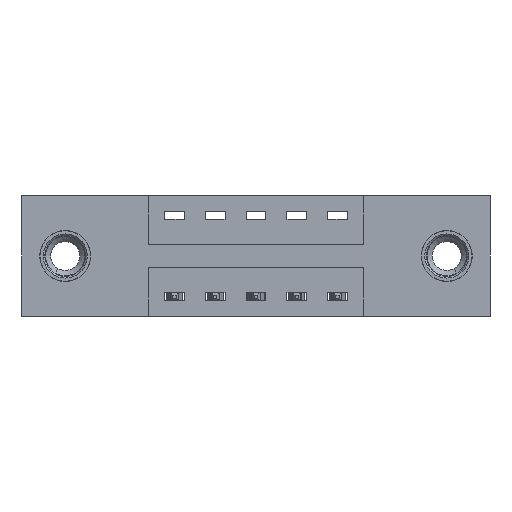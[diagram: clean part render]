
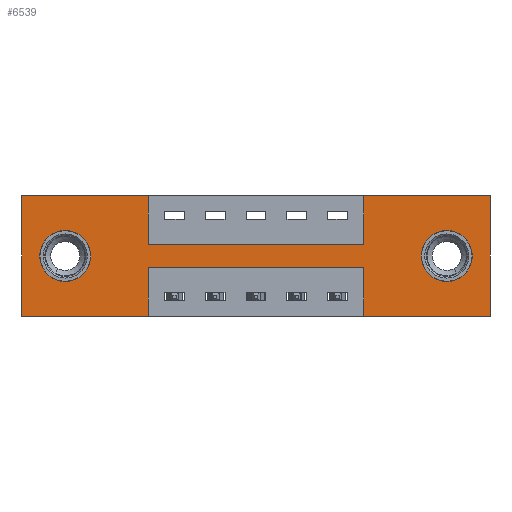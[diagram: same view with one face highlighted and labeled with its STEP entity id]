
A CAD part, front view. The second image highlights one B-rep face of the part: STEP entity #6539.
In plain terms, the highlighted planar face has unit normal (0, -1, 0).
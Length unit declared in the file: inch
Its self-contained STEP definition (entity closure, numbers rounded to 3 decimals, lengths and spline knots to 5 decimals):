
#58 = DIRECTION ( 'NONE',  ( 0., 1., 0. ) ) ;
#68 = LINE ( 'NONE', #8705, #10293 ) ;
#119 = VERTEX_POINT ( 'NONE', #5706 ) ;
#199 = ORIENTED_EDGE ( 'NONE', *, *, #5294, .T. ) ;
#257 = CIRCLE ( 'NONE', #3905, 0.078 ) ;
#302 = LINE ( 'NONE', #12804, #4380 ) ;
#514 = CIRCLE ( 'NONE', #6808, 0.078 ) ;
#545 = CARTESIAN_POINT ( 'NONE',  ( 0.3875, 0., -0.15 ) ) ;
#582 = EDGE_CURVE ( 'NONE', #119, #5072, #11572, .T. ) ;
#781 = VERTEX_POINT ( 'NONE', #3629 ) ;
#917 = CARTESIAN_POINT ( 'NONE',  ( 0.3875, 0., -0.15 ) ) ;
#975 = VECTOR ( 'NONE', #1886, 39.37008 ) ;
#1065 = VECTOR ( 'NONE', #10055, 39.37008 ) ;
#1067 = PLANE ( 'NONE',  #12464 ) ;
#1289 = LINE ( 'NONE', #8876, #2550 ) ;
#1296 = VERTEX_POINT ( 'NONE', #917 ) ;
#1305 = CARTESIAN_POINT ( 'NONE',  ( 0.3875, 0., 0. ) ) ;
#1380 = EDGE_LOOP ( 'NONE', ( #10732, #6123 ) ) ;
#1433 = ORIENTED_EDGE ( 'NONE', *, *, #582, .F. ) ;
#1445 = CARTESIAN_POINT ( 'NONE',  ( 1.3025, 0., -0.107 ) ) ;
#1469 = DIRECTION ( 'NONE',  ( 1., 0., 0. ) ) ;
#1517 = VERTEX_POINT ( 'NONE', #2110 ) ;
#1704 = CARTESIAN_POINT ( 'NONE',  ( 0., 0., 0. ) ) ;
#1751 = VECTOR ( 'NONE', #12090, 39.37008 ) ;
#1886 = DIRECTION ( 'NONE',  ( -1., 0., 0. ) ) ;
#1966 = ORIENTED_EDGE ( 'NONE', *, *, #2971, .F. ) ;
#1979 = CARTESIAN_POINT ( 'NONE',  ( 1.0475, 0., -0.15 ) ) ;
#2042 = VECTOR ( 'NONE', #8438, 39.37008 ) ;
#2110 = CARTESIAN_POINT ( 'NONE',  ( 1.3025, 0., -0.263 ) ) ;
#2323 = LINE ( 'NONE', #7987, #1065 ) ;
#2514 = LINE ( 'NONE', #545, #4100 ) ;
#2535 = VECTOR ( 'NONE', #4720, 39.37008 ) ;
#2550 = VECTOR ( 'NONE', #8923, 39.37008 ) ;
#2814 = EDGE_CURVE ( 'NONE', #9229, #6788, #2323, .T. ) ;
#2895 = EDGE_CURVE ( 'NONE', #12472, #7418, #257, .T. ) ;
#2971 = EDGE_CURVE ( 'NONE', #781, #9229, #11446, .T. ) ;
#3018 = DIRECTION ( 'NONE',  ( 0., 0., -1. ) ) ;
#3120 = VERTEX_POINT ( 'NONE', #1979 ) ;
#3123 = EDGE_LOOP ( 'NONE', ( #199, #5815 ) ) ;
#3542 = DIRECTION ( 'NONE',  ( 0., 0., 1. ) ) ;
#3629 = CARTESIAN_POINT ( 'NONE',  ( 0.3875, 0., -0.22 ) ) ;
#3746 = ORIENTED_EDGE ( 'NONE', *, *, #6496, .F. ) ;
#3786 = VECTOR ( 'NONE', #12459, 39.37008 ) ;
#3905 = AXIS2_PLACEMENT_3D ( 'NONE', #3908, #58, #9919 ) ;
#3908 = CARTESIAN_POINT ( 'NONE',  ( 0.1325, 0., -0.185 ) ) ;
#4011 = CARTESIAN_POINT ( 'NONE',  ( 0., 0., -0.37 ) ) ;
#4100 = VECTOR ( 'NONE', #1469, 39.37008 ) ;
#4112 = ORIENTED_EDGE ( 'NONE', *, *, #6840, .F. ) ;
#4281 = ORIENTED_EDGE ( 'NONE', *, *, #10582, .F. ) ;
#4380 = VECTOR ( 'NONE', #9010, 39.37008 ) ;
#4396 = CARTESIAN_POINT ( 'NONE',  ( 1.0475, 0., -0.22 ) ) ;
#4534 = CARTESIAN_POINT ( 'NONE',  ( 0.1325, 0., -0.185 ) ) ;
#4720 = DIRECTION ( 'NONE',  ( 0., 0., 1. ) ) ;
#4751 = ORIENTED_EDGE ( 'NONE', *, *, #6354, .F. ) ;
#4925 = CARTESIAN_POINT ( 'NONE',  ( 1.3025, 0., -0.185 ) ) ;
#4954 = EDGE_CURVE ( 'NONE', #1517, #7300, #10635, .T. ) ;
#5072 = VERTEX_POINT ( 'NONE', #4396 ) ;
#5158 = CARTESIAN_POINT ( 'NONE',  ( 0., 0., 0. ) ) ;
#5183 = LINE ( 'NONE', #11696, #2535 ) ;
#5198 = FACE_BOUND ( 'NONE', #1380, .T. ) ;
#5199 = DIRECTION ( 'NONE',  ( 0., 0., -1. ) ) ;
#5294 = EDGE_CURVE ( 'NONE', #7300, #1517, #514, .T. ) ;
#5363 = ORIENTED_EDGE ( 'NONE', *, *, #5824, .F. ) ;
#5441 = CARTESIAN_POINT ( 'NONE',  ( 0.3875, 0., -0.37 ) ) ;
#5706 = CARTESIAN_POINT ( 'NONE',  ( 1.0475, 0., -0.37 ) ) ;
#5815 = ORIENTED_EDGE ( 'NONE', *, *, #4954, .T. ) ;
#5824 = EDGE_CURVE ( 'NONE', #12373, #8103, #68, .T. ) ;
#5859 = VECTOR ( 'NONE', #5199, 39.37008 ) ;
#6123 = ORIENTED_EDGE ( 'NONE', *, *, #2895, .T. ) ;
#6354 = EDGE_CURVE ( 'NONE', #8103, #119, #11864, .T. ) ;
#6496 = EDGE_CURVE ( 'NONE', #9581, #1296, #1289, .T. ) ;
#6539 = ADVANCED_FACE ( 'NONE', ( #9507, #5198, #9838 ), #1067, .T. ) ;
#6545 = DIRECTION ( 'NONE',  ( 0., 1., 0. ) ) ;
#6579 = DIRECTION ( 'NONE',  ( 0., 0., -1. ) ) ;
#6753 = EDGE_CURVE ( 'NONE', #6788, #12487, #5183, .T. ) ;
#6788 = VERTEX_POINT ( 'NONE', #8521 ) ;
#6808 = AXIS2_PLACEMENT_3D ( 'NONE', #11784, #9593, #7630 ) ;
#6829 = CARTESIAN_POINT ( 'NONE',  ( 0., 0., -0.37 ) ) ;
#6840 = EDGE_CURVE ( 'NONE', #12487, #9581, #11345, .T. ) ;
#6937 = CARTESIAN_POINT ( 'NONE',  ( 1.435, 0., 0. ) ) ;
#7300 = VERTEX_POINT ( 'NONE', #1445 ) ;
#7341 = DIRECTION ( 'NONE',  ( 0., 0., 1. ) ) ;
#7393 = CARTESIAN_POINT ( 'NONE',  ( 1.0475, 0., 0. ) ) ;
#7418 = VERTEX_POINT ( 'NONE', #8913 ) ;
#7498 = ORIENTED_EDGE ( 'NONE', *, *, #6753, .F. ) ;
#7612 = VERTEX_POINT ( 'NONE', #10542 ) ;
#7630 = DIRECTION ( 'NONE',  ( 0., 0., -1. ) ) ;
#7633 = ORIENTED_EDGE ( 'NONE', *, *, #10888, .F. ) ;
#7859 = VECTOR ( 'NONE', #3542, 39.37008 ) ;
#7868 = AXIS2_PLACEMENT_3D ( 'NONE', #4534, #6545, #7341 ) ;
#7987 = CARTESIAN_POINT ( 'NONE',  ( 0., 0., -0.37 ) ) ;
#8103 = VERTEX_POINT ( 'NONE', #10411 ) ;
#8438 = DIRECTION ( 'NONE',  ( 0., 0., 1. ) ) ;
#8521 = CARTESIAN_POINT ( 'NONE',  ( 0., 0., -0.37 ) ) ;
#8705 = CARTESIAN_POINT ( 'NONE',  ( 1.435, 0., 0. ) ) ;
#8876 = CARTESIAN_POINT ( 'NONE',  ( 0.3875, 0., 0. ) ) ;
#8883 = LINE ( 'NONE', #9454, #3786 ) ;
#8913 = CARTESIAN_POINT ( 'NONE',  ( 0.1325, 0., -0.107 ) ) ;
#8923 = DIRECTION ( 'NONE',  ( 0., 0., -1. ) ) ;
#9005 = DIRECTION ( 'NONE',  ( 0., -1., 0. ) ) ;
#9010 = DIRECTION ( 'NONE',  ( 1., 0., 0. ) ) ;
#9139 = ORIENTED_EDGE ( 'NONE', *, *, #2814, .F. ) ;
#9208 = ORIENTED_EDGE ( 'NONE', *, *, #10073, .F. ) ;
#9229 = VERTEX_POINT ( 'NONE', #5441 ) ;
#9365 = CARTESIAN_POINT ( 'NONE',  ( 1.0475, 0., -0.37 ) ) ;
#9454 = CARTESIAN_POINT ( 'NONE',  ( 0.3875, 0., -0.22 ) ) ;
#9489 = CIRCLE ( 'NONE', #7868, 0.078 ) ;
#9507 = FACE_BOUND ( 'NONE', #3123, .T. ) ;
#9581 = VERTEX_POINT ( 'NONE', #1305 ) ;
#9593 = DIRECTION ( 'NONE',  ( 0., 1., 0. ) ) ;
#9721 = AXIS2_PLACEMENT_3D ( 'NONE', #4925, #11848, #3018 ) ;
#9838 = FACE_OUTER_BOUND ( 'NONE', #12853, .T. ) ;
#9919 = DIRECTION ( 'NONE',  ( 0., 0., 1. ) ) ;
#10006 = DIRECTION ( 'NONE',  ( 0., 0., -1. ) ) ;
#10055 = DIRECTION ( 'NONE',  ( -1., 0., 0. ) ) ;
#10073 = EDGE_CURVE ( 'NONE', #5072, #781, #8883, .T. ) ;
#10293 = VECTOR ( 'NONE', #6579, 39.37008 ) ;
#10411 = CARTESIAN_POINT ( 'NONE',  ( 1.435, 0., -0.37 ) ) ;
#10542 = CARTESIAN_POINT ( 'NONE',  ( 1.0475, 0., 0. ) ) ;
#10582 = EDGE_CURVE ( 'NONE', #1296, #3120, #2514, .T. ) ;
#10635 = CIRCLE ( 'NONE', #9721, 0.078 ) ;
#10732 = ORIENTED_EDGE ( 'NONE', *, *, #11133, .T. ) ;
#10888 = EDGE_CURVE ( 'NONE', #7612, #12373, #302, .T. ) ;
#11077 = CARTESIAN_POINT ( 'NONE',  ( 0.3875, 0., -0.37 ) ) ;
#11133 = EDGE_CURVE ( 'NONE', #7418, #12472, #9489, .T. ) ;
#11345 = LINE ( 'NONE', #5158, #1751 ) ;
#11446 = LINE ( 'NONE', #11077, #5859 ) ;
#11494 = LINE ( 'NONE', #7393, #2042 ) ;
#11572 = LINE ( 'NONE', #9365, #7859 ) ;
#11696 = CARTESIAN_POINT ( 'NONE',  ( 0., 0., 0. ) ) ;
#11784 = CARTESIAN_POINT ( 'NONE',  ( 1.3025, 0., -0.185 ) ) ;
#11848 = DIRECTION ( 'NONE',  ( 0., 1., 0. ) ) ;
#11864 = LINE ( 'NONE', #6829, #975 ) ;
#12090 = DIRECTION ( 'NONE',  ( 1., 0., 0. ) ) ;
#12229 = ORIENTED_EDGE ( 'NONE', *, *, #12664, .F. ) ;
#12373 = VERTEX_POINT ( 'NONE', #6937 ) ;
#12459 = DIRECTION ( 'NONE',  ( -1., 0., 0. ) ) ;
#12464 = AXIS2_PLACEMENT_3D ( 'NONE', #4011, #9005, #10006 ) ;
#12472 = VERTEX_POINT ( 'NONE', #12540 ) ;
#12487 = VERTEX_POINT ( 'NONE', #1704 ) ;
#12540 = CARTESIAN_POINT ( 'NONE',  ( 0.1325, 0., -0.263 ) ) ;
#12664 = EDGE_CURVE ( 'NONE', #3120, #7612, #11494, .T. ) ;
#12804 = CARTESIAN_POINT ( 'NONE',  ( 0., 0., 0. ) ) ;
#12853 = EDGE_LOOP ( 'NONE', ( #1966, #9208, #1433, #4751, #5363, #7633, #12229, #4281, #3746, #4112, #7498, #9139 ) ) ;
